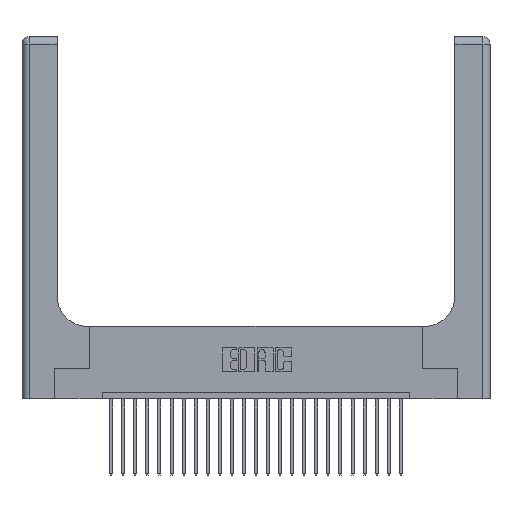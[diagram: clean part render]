
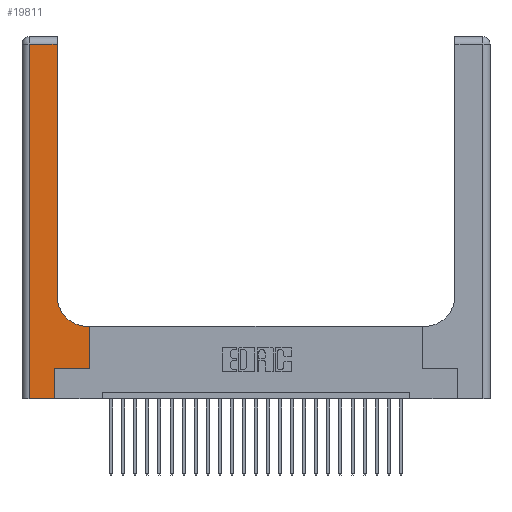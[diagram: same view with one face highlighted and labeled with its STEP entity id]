
A CAD part, top view. The second image highlights one B-rep face of the part: STEP entity #19811.
In plain terms, the highlighted planar face has unit normal (0, 0, 1).
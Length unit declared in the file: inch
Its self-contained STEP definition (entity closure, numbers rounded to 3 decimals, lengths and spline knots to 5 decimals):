
#26333 = DIRECTION ( 'NONE',  ( -1., 0., 0. ) ) ;
#66 = CARTESIAN_POINT ( 'NONE',  ( 0., 3., 0.37 ) ) ;
#70 = EDGE_CURVE ( 'NONE', #10660, #22197, #2129, .T. ) ;
#229 = DIRECTION ( 'NONE',  ( 0., 0., -1. ) ) ;
#656 = LINE ( 'NONE', #3067, #14304 ) ;
#1336 = CARTESIAN_POINT ( 'NONE',  ( 0.2915, 2.94, 0.37 ) ) ;
#1420 = VERTEX_POINT ( 'NONE', #18000 ) ;
#1520 = VECTOR ( 'NONE', #19469, 39.37008 ) ;
#2082 = VERTEX_POINT ( 'NONE', #7738 ) ;
#2129 = LINE ( 'NONE', #5799, #16437 ) ;
#3067 = CARTESIAN_POINT ( 'NONE',  ( 0.2915, 3., 0.37 ) ) ;
#3519 = CARTESIAN_POINT ( 'NONE',  ( 0.2915, 0.85, 0.37 ) ) ;
#4145 = LINE ( 'NONE', #8135, #17475 ) ;
#4219 = AXIS2_PLACEMENT_3D ( 'NONE', #66, #229, #20461 ) ;
#4254 = EDGE_CURVE ( 'NONE', #23668, #1420, #4145, .T. ) ;
#4353 = VECTOR ( 'NONE', #13051, 39.37008 ) ;
#4479 = ORIENTED_EDGE ( 'NONE', *, *, #26046, .T. ) ;
#4577 = DIRECTION ( 'NONE',  ( 0., -1., 0. ) ) ;
#5009 = VERTEX_POINT ( 'NONE', #16957 ) ;
#5161 = VERTEX_POINT ( 'NONE', #1336 ) ;
#5799 = CARTESIAN_POINT ( 'NONE',  ( 0.269, 0., 0.37 ) ) ;
#5872 = DIRECTION ( 'NONE',  ( -1., 0., 0. ) ) ;
#6200 = LINE ( 'NONE', #14094, #19181 ) ;
#6283 = CARTESIAN_POINT ( 'NONE',  ( 0.06, 3., 0.37 ) ) ;
#6313 = LINE ( 'NONE', #13598, #1520 ) ;
#6372 = DIRECTION ( 'NONE',  ( 0., 1., 0. ) ) ;
#7216 = ORIENTED_EDGE ( 'NONE', *, *, #23122, .T. ) ;
#7239 = ORIENTED_EDGE ( 'NONE', *, *, #70, .T. ) ;
#7738 = CARTESIAN_POINT ( 'NONE',  ( 0.06, 0., 0.37 ) ) ;
#8119 = EDGE_LOOP ( 'NONE', ( #14342, #25219, #17706, #4479, #7239, #7216, #9657, #9983, #15431 ) ) ;
#8135 = CARTESIAN_POINT ( 'NONE',  ( 0.5585, 0.25, 0.37 ) ) ;
#8491 = LINE ( 'NONE', #11968, #10728 ) ;
#8504 = CARTESIAN_POINT ( 'NONE',  ( 0.269, 0.25, 0.37 ) ) ;
#8674 = EDGE_CURVE ( 'NONE', #16794, #5161, #656, .T. ) ;
#9657 = ORIENTED_EDGE ( 'NONE', *, *, #4254, .T. ) ;
#9983 = ORIENTED_EDGE ( 'NONE', *, *, #12669, .T. ) ;
#10660 = VERTEX_POINT ( 'NONE', #11217 ) ;
#10728 = VECTOR ( 'NONE', #26333, 39.37008 ) ;
#11217 = CARTESIAN_POINT ( 'NONE',  ( 0.269, 0., 0.37 ) ) ;
#11942 = EDGE_CURVE ( 'NONE', #25981, #2082, #12246, .T. ) ;
#11968 = CARTESIAN_POINT ( 'NONE',  ( 0., 2.94, 0.37 ) ) ;
#12246 = LINE ( 'NONE', #6283, #15782 ) ;
#12669 = EDGE_CURVE ( 'NONE', #1420, #5009, #6200, .T. ) ;
#12819 = FACE_OUTER_BOUND ( 'NONE', #8119, .T. ) ;
#13051 = DIRECTION ( 'NONE',  ( 1., 0., 0. ) ) ;
#13598 = CARTESIAN_POINT ( 'NONE',  ( 0.269, 0.25, 0.37 ) ) ;
#14094 = CARTESIAN_POINT ( 'NONE',  ( 0.2915, 0.6, 0.37 ) ) ;
#14304 = VECTOR ( 'NONE', #19123, 39.37008 ) ;
#14342 = ORIENTED_EDGE ( 'NONE', *, *, #8674, .T. ) ;
#15431 = ORIENTED_EDGE ( 'NONE', *, *, #16041, .T. ) ;
#15782 = VECTOR ( 'NONE', #4577, 39.37008 ) ;
#16041 = EDGE_CURVE ( 'NONE', #5009, #16794, #26043, .T. ) ;
#16437 = VECTOR ( 'NONE', #18002, 39.37008 ) ;
#16794 = VERTEX_POINT ( 'NONE', #3519 ) ;
#16957 = CARTESIAN_POINT ( 'NONE',  ( 0.5415, 0.6, 0.37 ) ) ;
#17060 = LINE ( 'NONE', #25293, #4353 ) ;
#17245 = CARTESIAN_POINT ( 'NONE',  ( 0.06, 2.94, 0.37 ) ) ;
#17475 = VECTOR ( 'NONE', #6372, 39.37008 ) ;
#17706 = ORIENTED_EDGE ( 'NONE', *, *, #11942, .T. ) ;
#18000 = CARTESIAN_POINT ( 'NONE',  ( 0.5585, 0.6, 0.37 ) ) ;
#18002 = DIRECTION ( 'NONE',  ( 0., 1., 0. ) ) ;
#19123 = DIRECTION ( 'NONE',  ( 0., 1., 0. ) ) ;
#19181 = VECTOR ( 'NONE', #5872, 39.37008 ) ;
#19469 = DIRECTION ( 'NONE',  ( 1., 0., 0. ) ) ;
#19811 = ADVANCED_FACE ( 'NONE', ( #12819 ), #24532, .F. ) ;
#20461 = DIRECTION ( 'NONE',  ( -1., 0., 0. ) ) ;
#20955 = DIRECTION ( 'NONE',  ( 1., 0., 0. ) ) ;
#21213 = DIRECTION ( 'NONE',  ( 0., 0., -1. ) ) ;
#22197 = VERTEX_POINT ( 'NONE', #8504 ) ;
#23122 = EDGE_CURVE ( 'NONE', #22197, #23668, #6313, .T. ) ;
#23160 = AXIS2_PLACEMENT_3D ( 'NONE', #24935, #21213, #20955 ) ;
#23668 = VERTEX_POINT ( 'NONE', #23685 ) ;
#23685 = CARTESIAN_POINT ( 'NONE',  ( 0.5585, 0.25, 0.37 ) ) ;
#23774 = EDGE_CURVE ( 'NONE', #5161, #25981, #8491, .T. ) ;
#24532 = PLANE ( 'NONE',  #4219 ) ;
#24935 = CARTESIAN_POINT ( 'NONE',  ( 0.5415, 0.85, 0.37 ) ) ;
#25219 = ORIENTED_EDGE ( 'NONE', *, *, #23774, .T. ) ;
#25293 = CARTESIAN_POINT ( 'NONE',  ( 0., 0., 0.37 ) ) ;
#25981 = VERTEX_POINT ( 'NONE', #17245 ) ;
#26043 = CIRCLE ( 'NONE', #23160, 0.25 ) ;
#26046 = EDGE_CURVE ( 'NONE', #2082, #10660, #17060, .T. ) ;
